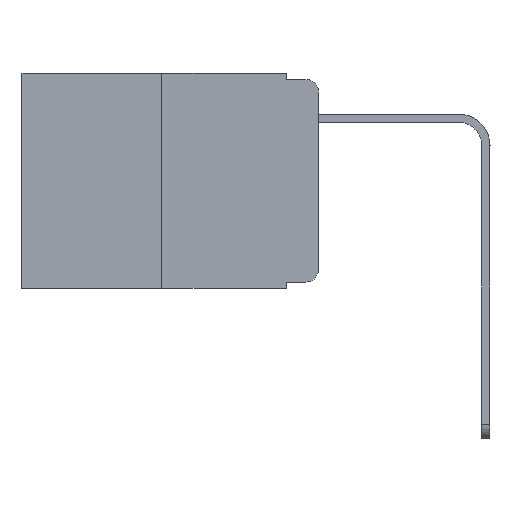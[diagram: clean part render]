
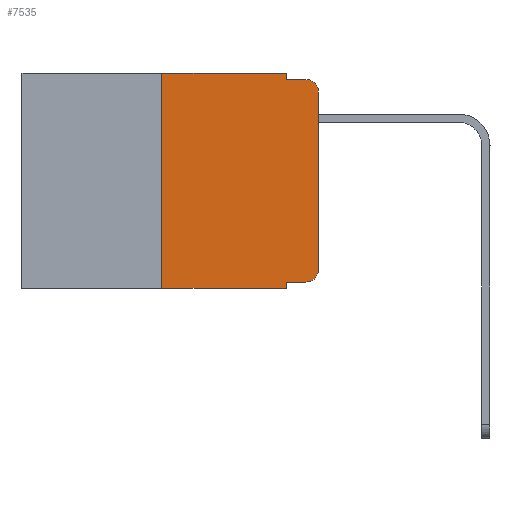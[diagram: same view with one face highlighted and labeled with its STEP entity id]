
A CAD part, left-side view. The second image highlights one B-rep face of the part: STEP entity #7535.
In plain terms, the highlighted planar face has unit normal (-1, 0, 0).
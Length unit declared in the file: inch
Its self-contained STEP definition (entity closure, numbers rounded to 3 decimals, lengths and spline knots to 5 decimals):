
#707 = ORIENTED_EDGE ( 'NONE', *, *, #14124, .T. ) ;
#771 = CARTESIAN_POINT ( 'NONE',  ( 0., 0.051, -0.333 ) ) ;
#784 = ORIENTED_EDGE ( 'NONE', *, *, #19185, .T. ) ;
#1140 = ORIENTED_EDGE ( 'NONE', *, *, #18992, .T. ) ;
#1205 = CARTESIAN_POINT ( 'NONE',  ( 0., 0.051, 0. ) ) ;
#2202 = DIRECTION ( 'NONE',  ( 0., -1., 0. ) ) ;
#2227 = CARTESIAN_POINT ( 'NONE',  ( 0., 0.051, -0.01 ) ) ;
#2546 = ORIENTED_EDGE ( 'NONE', *, *, #7720, .F. ) ;
#3120 = VERTEX_POINT ( 'NONE', #17006 ) ;
#3158 = VECTOR ( 'NONE', #5276, 39.37008 ) ;
#3463 = ORIENTED_EDGE ( 'NONE', *, *, #14154, .T. ) ;
#3492 = VERTEX_POINT ( 'NONE', #13625 ) ;
#3584 = VERTEX_POINT ( 'NONE', #18463 ) ;
#3694 = CARTESIAN_POINT ( 'NONE',  ( 0., 0.051, -0.333 ) ) ;
#3819 = VECTOR ( 'NONE', #2202, 39.37008 ) ;
#4067 = LINE ( 'NONE', #2227, #3158 ) ;
#4074 = DIRECTION ( 'NONE',  ( 0., 0., -1. ) ) ;
#4229 = CIRCLE ( 'NONE', #13285, 0.02 ) ;
#4239 = VERTEX_POINT ( 'NONE', #3694 ) ;
#4260 = CARTESIAN_POINT ( 'NONE',  ( 0., 0.02, -0.03 ) ) ;
#4516 = VECTOR ( 'NONE', #16139, 39.37008 ) ;
#4553 = DIRECTION ( 'NONE',  ( 0., -1., 0. ) ) ;
#5276 = DIRECTION ( 'NONE',  ( 0., -1., 0. ) ) ;
#5538 = CARTESIAN_POINT ( 'NONE',  ( 0., 0.051, -0.343 ) ) ;
#6046 = AXIS2_PLACEMENT_3D ( 'NONE', #8362, #12731, #15678 ) ;
#6400 = FACE_OUTER_BOUND ( 'NONE', #15593, .T. ) ;
#6424 = CIRCLE ( 'NONE', #10314, 0.02 ) ;
#6590 = CARTESIAN_POINT ( 'NONE',  ( 0., 0.02, -0.333 ) ) ;
#6720 = VERTEX_POINT ( 'NONE', #9369 ) ;
#7265 = CARTESIAN_POINT ( 'NONE',  ( 0., 0.051, 0. ) ) ;
#7353 = DIRECTION ( 'NONE',  ( 0., 0., -1. ) ) ;
#7465 = EDGE_CURVE ( 'NONE', #6720, #18748, #15889, .T. ) ;
#7535 = ADVANCED_FACE ( 'NONE', ( #6400 ), #14170, .F. ) ;
#7603 = EDGE_CURVE ( 'NONE', #6720, #8877, #17318, .T. ) ;
#7720 = EDGE_CURVE ( 'NONE', #4239, #18748, #18927, .T. ) ;
#8362 = CARTESIAN_POINT ( 'NONE',  ( 0., 0.473, 0. ) ) ;
#8527 = ORIENTED_EDGE ( 'NONE', *, *, #7465, .T. ) ;
#8877 = VERTEX_POINT ( 'NONE', #16987 ) ;
#8953 = VECTOR ( 'NONE', #12099, 39.37008 ) ;
#9183 = VECTOR ( 'NONE', #12992, 39.37008 ) ;
#9369 = CARTESIAN_POINT ( 'NONE',  ( 0., 0.25, -0.343 ) ) ;
#10274 = DIRECTION ( 'NONE',  ( 0., 0., -1. ) ) ;
#10314 = AXIS2_PLACEMENT_3D ( 'NONE', #17532, #11662, #4074 ) ;
#10331 = ORIENTED_EDGE ( 'NONE', *, *, #17548, .F. ) ;
#11351 = CARTESIAN_POINT ( 'NONE',  ( 0., 0.051, 0. ) ) ;
#11662 = DIRECTION ( 'NONE',  ( -1., 0., 0. ) ) ;
#11706 = LINE ( 'NONE', #771, #3819 ) ;
#12099 = DIRECTION ( 'NONE',  ( 0., 0., 1. ) ) ;
#12659 = ORIENTED_EDGE ( 'NONE', *, *, #18624, .F. ) ;
#12731 = DIRECTION ( 'NONE',  ( 1., 0., 0. ) ) ;
#12850 = VERTEX_POINT ( 'NONE', #11351 ) ;
#12969 = ORIENTED_EDGE ( 'NONE', *, *, #7603, .F. ) ;
#12992 = DIRECTION ( 'NONE',  ( 0., 0., -1. ) ) ;
#13187 = CARTESIAN_POINT ( 'NONE',  ( 0., 0.25, 0. ) ) ;
#13285 = AXIS2_PLACEMENT_3D ( 'NONE', #4260, #14628, #7353 ) ;
#13372 = LINE ( 'NONE', #16456, #16911 ) ;
#13625 = CARTESIAN_POINT ( 'NONE',  ( 0., 0.051, -0.01 ) ) ;
#13916 = CARTESIAN_POINT ( 'NONE',  ( 0., 0.473, -0.343 ) ) ;
#14094 = VECTOR ( 'NONE', #10274, 39.37008 ) ;
#14124 = EDGE_CURVE ( 'NONE', #15652, #3584, #6424, .T. ) ;
#14154 = EDGE_CURVE ( 'NONE', #3120, #18513, #4229, .T. ) ;
#14170 = PLANE ( 'NONE',  #6046 ) ;
#14628 = DIRECTION ( 'NONE',  ( -1., 0., 0. ) ) ;
#15425 = DIRECTION ( 'NONE',  ( 0., -1., 0. ) ) ;
#15593 = EDGE_LOOP ( 'NONE', ( #1140, #3463, #12659, #10331, #18804, #12969, #8527, #2546, #784, #707 ) ) ;
#15652 = VERTEX_POINT ( 'NONE', #6590 ) ;
#15676 = LINE ( 'NONE', #18046, #8953 ) ;
#15678 = DIRECTION ( 'NONE',  ( 0., 0., -1. ) ) ;
#15889 = LINE ( 'NONE', #13916, #16631 ) ;
#16139 = DIRECTION ( 'NONE',  ( 0., 0., 1. ) ) ;
#16456 = CARTESIAN_POINT ( 'NONE',  ( 0., 0.473, 0. ) ) ;
#16631 = VECTOR ( 'NONE', #15425, 39.37008 ) ;
#16911 = VECTOR ( 'NONE', #4553, 39.37008 ) ;
#16987 = CARTESIAN_POINT ( 'NONE',  ( 0., 0.25, 0. ) ) ;
#17006 = CARTESIAN_POINT ( 'NONE',  ( 0., 0., -0.03 ) ) ;
#17170 = LINE ( 'NONE', #1205, #14094 ) ;
#17318 = LINE ( 'NONE', #13187, #4516 ) ;
#17532 = CARTESIAN_POINT ( 'NONE',  ( 0., 0.02, -0.313 ) ) ;
#17548 = EDGE_CURVE ( 'NONE', #12850, #3492, #17170, .T. ) ;
#18046 = CARTESIAN_POINT ( 'NONE',  ( 0., 0., 0. ) ) ;
#18323 = EDGE_CURVE ( 'NONE', #8877, #12850, #13372, .T. ) ;
#18333 = CARTESIAN_POINT ( 'NONE',  ( 0., 0.02, -0.01 ) ) ;
#18463 = CARTESIAN_POINT ( 'NONE',  ( 0., 0., -0.313 ) ) ;
#18513 = VERTEX_POINT ( 'NONE', #18333 ) ;
#18624 = EDGE_CURVE ( 'NONE', #3492, #18513, #4067, .T. ) ;
#18748 = VERTEX_POINT ( 'NONE', #5538 ) ;
#18804 = ORIENTED_EDGE ( 'NONE', *, *, #18323, .F. ) ;
#18927 = LINE ( 'NONE', #7265, #9183 ) ;
#18992 = EDGE_CURVE ( 'NONE', #3584, #3120, #15676, .T. ) ;
#19185 = EDGE_CURVE ( 'NONE', #4239, #15652, #11706, .T. ) ;
